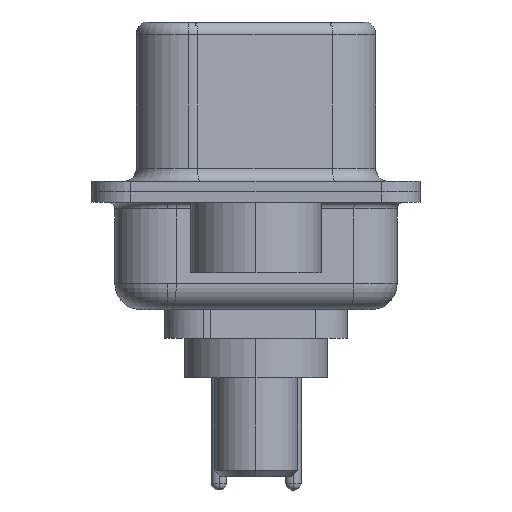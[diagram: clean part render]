
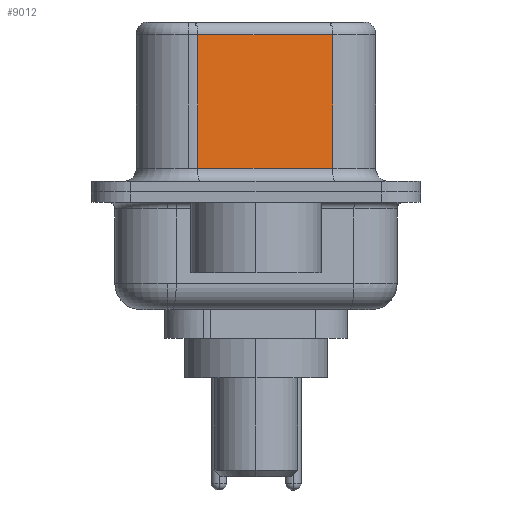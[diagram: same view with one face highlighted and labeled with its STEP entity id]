
A CAD part, left-side view. The second image highlights one B-rep face of the part: STEP entity #9012.
In plain terms, the highlighted planar face has unit normal (-0.985, -0.174, 0).
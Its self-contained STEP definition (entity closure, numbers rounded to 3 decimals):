
#52 = CARTESIAN_POINT ( 'NONE',  ( 4.58, -2.927, 6.52 ) ) ;
#172 = VECTOR ( 'NONE', #18288, 1000. ) ;
#1988 = DIRECTION ( 'NONE',  ( -0.174, 0.985, 0. ) ) ;
#3527 = EDGE_CURVE ( 'NONE', #4718, #17401, #8334, .T. ) ;
#4274 = VERTEX_POINT ( 'NONE', #20081 ) ;
#4592 = EDGE_CURVE ( 'NONE', #7412, #4718, #12599, .T. ) ;
#4718 = VERTEX_POINT ( 'NONE', #19297 ) ;
#4769 = CARTESIAN_POINT ( 'NONE',  ( 4.58, -2.927, 0.9 ) ) ;
#5097 = VECTOR ( 'NONE', #23063, 1000. ) ;
#5749 = EDGE_CURVE ( 'NONE', #4274, #17401, #14069, .T. ) ;
#6406 = EDGE_LOOP ( 'NONE', ( #22911, #14335, #11446, #9639 ) ) ;
#7405 = DIRECTION ( 'NONE',  ( 0., 0., -1. ) ) ;
#7412 = VERTEX_POINT ( 'NONE', #22744 ) ;
#7444 = CARTESIAN_POINT ( 'NONE',  ( 4.58, -2.927, 6.52 ) ) ;
#8334 = LINE ( 'NONE', #4769, #14642 ) ;
#8399 = CARTESIAN_POINT ( 'NONE',  ( 4.58, -2.927, 6.02 ) ) ;
#8413 = DIRECTION ( 'NONE',  ( 0.174, -0.985, 0. ) ) ;
#9012 = ADVANCED_FACE ( 'NONE', ( #14528 ), #22428, .F. ) ;
#9639 = ORIENTED_EDGE ( 'NONE', *, *, #3527, .T. ) ;
#10008 = CARTESIAN_POINT ( 'NONE',  ( 4.58, -2.927, 0.9 ) ) ;
#11446 = ORIENTED_EDGE ( 'NONE', *, *, #4592, .T. ) ;
#12069 = CARTESIAN_POINT ( 'NONE',  ( 3.67, 2.233, 6.52 ) ) ;
#12599 = LINE ( 'NONE', #12069, #17490 ) ;
#14069 = LINE ( 'NONE', #7444, #172 ) ;
#14335 = ORIENTED_EDGE ( 'NONE', *, *, #21772, .T. ) ;
#14528 = FACE_OUTER_BOUND ( 'NONE', #6406, .T. ) ;
#14642 = VECTOR ( 'NONE', #8413, 1000. ) ;
#17401 = VERTEX_POINT ( 'NONE', #10008 ) ;
#17490 = VECTOR ( 'NONE', #7405, 1000. ) ;
#18288 = DIRECTION ( 'NONE',  ( 0., 0., -1. ) ) ;
#19297 = CARTESIAN_POINT ( 'NONE',  ( 3.67, 2.233, 0.9 ) ) ;
#19513 = AXIS2_PLACEMENT_3D ( 'NONE', #52, #24231, #1988 ) ;
#20081 = CARTESIAN_POINT ( 'NONE',  ( 4.58, -2.927, 6.02 ) ) ;
#21772 = EDGE_CURVE ( 'NONE', #4274, #7412, #23654, .T. ) ;
#22428 = PLANE ( 'NONE',  #19513 ) ;
#22744 = CARTESIAN_POINT ( 'NONE',  ( 3.67, 2.233, 6.02 ) ) ;
#22911 = ORIENTED_EDGE ( 'NONE', *, *, #5749, .F. ) ;
#23063 = DIRECTION ( 'NONE',  ( -0.174, 0.985, 0. ) ) ;
#23654 = LINE ( 'NONE', #8399, #5097 ) ;
#24231 = DIRECTION ( 'NONE',  ( 0.985, 0.174, 0. ) ) ;
